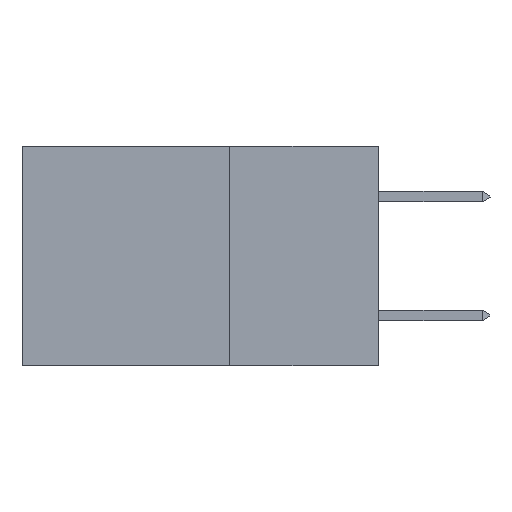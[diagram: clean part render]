
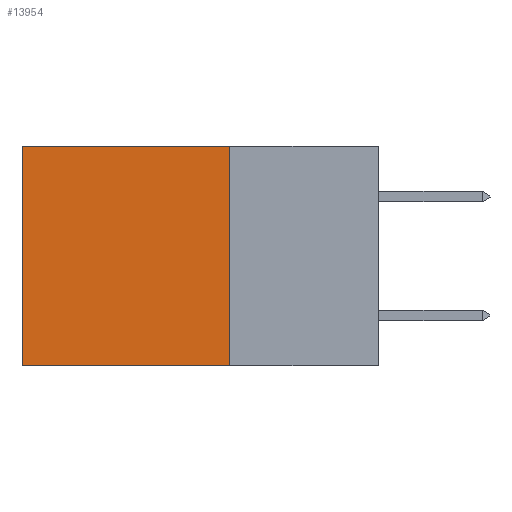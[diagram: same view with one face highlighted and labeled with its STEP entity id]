
A CAD part, left-side view. The second image highlights one B-rep face of the part: STEP entity #13954.
In plain terms, the highlighted planar face has unit normal (-1, 0, 0).
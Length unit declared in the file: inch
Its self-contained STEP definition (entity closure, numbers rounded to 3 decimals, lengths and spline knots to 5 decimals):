
#1152 = LINE ( 'NONE', #9246, #10701 ) ;
#1368 = LINE ( 'NONE', #10838, #6442 ) ;
#2329 = ORIENTED_EDGE ( 'NONE', *, *, #27881, .F. ) ;
#2370 = EDGE_CURVE ( 'NONE', #25232, #11385, #1368, .T. ) ;
#2403 = AXIS2_PLACEMENT_3D ( 'NONE', #6877, #22143, #9091 ) ;
#3383 = ORIENTED_EDGE ( 'NONE', *, *, #12190, .F. ) ;
#4320 = CARTESIAN_POINT ( 'NONE',  ( 0.298, 0.6, 0. ) ) ;
#4552 = CARTESIAN_POINT ( 'NONE',  ( 0.298, 0.25, 0. ) ) ;
#6092 = VERTEX_POINT ( 'NONE', #6741 ) ;
#6442 = VECTOR ( 'NONE', #9041, 39.37008 ) ;
#6741 = CARTESIAN_POINT ( 'NONE',  ( 0.298, 0.6, -0.37 ) ) ;
#6877 = CARTESIAN_POINT ( 'NONE',  ( 0.298, 0.25, 0. ) ) ;
#7888 = CARTESIAN_POINT ( 'NONE',  ( 0.298, 0.25, -0.37 ) ) ;
#8240 = CARTESIAN_POINT ( 'NONE',  ( 0.298, 0.6, 0. ) ) ;
#9041 = DIRECTION ( 'NONE',  ( 0., 1., 0. ) ) ;
#9091 = DIRECTION ( 'NONE',  ( 0., 0., -1. ) ) ;
#9246 = CARTESIAN_POINT ( 'NONE',  ( 0.298, 0.25, 0. ) ) ;
#9339 = VERTEX_POINT ( 'NONE', #7888 ) ;
#10567 = VECTOR ( 'NONE', #19096, 39.37008 ) ;
#10701 = VECTOR ( 'NONE', #11465, 39.37008 ) ;
#10838 = CARTESIAN_POINT ( 'NONE',  ( 0.298, 0.25, 0. ) ) ;
#11385 = VERTEX_POINT ( 'NONE', #4320 ) ;
#11465 = DIRECTION ( 'NONE',  ( 0., 0., -1. ) ) ;
#12190 = EDGE_CURVE ( 'NONE', #25232, #9339, #1152, .T. ) ;
#13564 = ORIENTED_EDGE ( 'NONE', *, *, #2370, .T. ) ;
#13954 = ADVANCED_FACE ( 'NONE', ( #17080 ), #17781, .F. ) ;
#15090 = CARTESIAN_POINT ( 'NONE',  ( 0.298, 0.25, -0.37 ) ) ;
#16564 = VECTOR ( 'NONE', #17249, 39.37008 ) ;
#17080 = FACE_OUTER_BOUND ( 'NONE', #26384, .T. ) ;
#17249 = DIRECTION ( 'NONE',  ( 0., 1., 0. ) ) ;
#17781 = PLANE ( 'NONE',  #2403 ) ;
#19096 = DIRECTION ( 'NONE',  ( 0., 0., -1. ) ) ;
#19252 = EDGE_CURVE ( 'NONE', #11385, #6092, #22141, .T. ) ;
#22141 = LINE ( 'NONE', #8240, #10567 ) ;
#22143 = DIRECTION ( 'NONE',  ( 1., 0., 0. ) ) ;
#23617 = ORIENTED_EDGE ( 'NONE', *, *, #19252, .T. ) ;
#25232 = VERTEX_POINT ( 'NONE', #4552 ) ;
#26384 = EDGE_LOOP ( 'NONE', ( #23617, #2329, #3383, #13564 ) ) ;
#27881 = EDGE_CURVE ( 'NONE', #9339, #6092, #27969, .T. ) ;
#27969 = LINE ( 'NONE', #15090, #16564 ) ;
